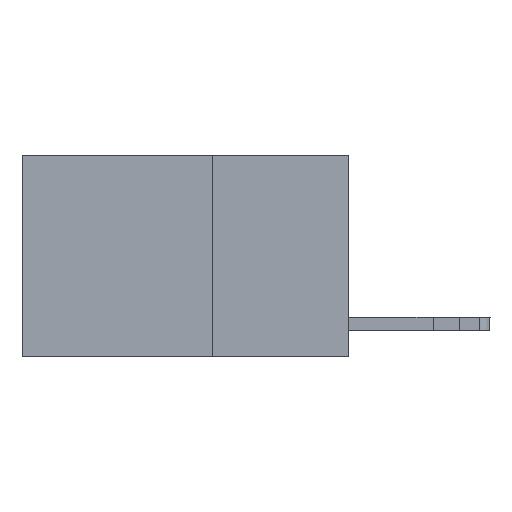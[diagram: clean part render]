
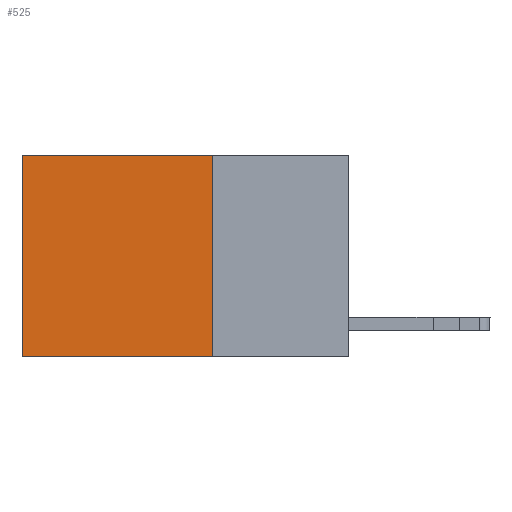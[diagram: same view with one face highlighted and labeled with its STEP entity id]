
A CAD part, left-side view. The second image highlights one B-rep face of the part: STEP entity #525.
In plain terms, the highlighted planar face has unit normal (-1, 0, 0).
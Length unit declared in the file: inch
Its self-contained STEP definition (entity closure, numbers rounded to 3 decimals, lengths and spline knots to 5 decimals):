
#215 = CARTESIAN_POINT ( 'NONE',  ( 0.2625, 0.6, -0.37 ) ) ;
#273 = VECTOR ( 'NONE', #13668, 39.37008 ) ;
#525 = ADVANCED_FACE ( 'NONE', ( #3201 ), #895, .F. ) ;
#894 = LINE ( 'NONE', #5625, #904 ) ;
#895 = PLANE ( 'NONE',  #9127 ) ;
#904 = VECTOR ( 'NONE', #4473, 39.37008 ) ;
#941 = EDGE_LOOP ( 'NONE', ( #10116, #12666, #1275, #1134 ) ) ;
#1053 = VERTEX_POINT ( 'NONE', #13430 ) ;
#1134 = ORIENTED_EDGE ( 'NONE', *, *, #11515, .T. ) ;
#1275 = ORIENTED_EDGE ( 'NONE', *, *, #5116, .F. ) ;
#1899 = CARTESIAN_POINT ( 'NONE',  ( 0.2625, 0.25, 0. ) ) ;
#3201 = FACE_OUTER_BOUND ( 'NONE', #941, .T. ) ;
#3376 = LINE ( 'NONE', #5924, #11583 ) ;
#3482 = VERTEX_POINT ( 'NONE', #215 ) ;
#3526 = EDGE_CURVE ( 'NONE', #1053, #3482, #3376, .T. ) ;
#4473 = DIRECTION ( 'NONE',  ( 0., 0., -1. ) ) ;
#5116 = EDGE_CURVE ( 'NONE', #12735, #12902, #894, .T. ) ;
#5625 = CARTESIAN_POINT ( 'NONE',  ( 0.2625, 0.25, 0. ) ) ;
#5765 = DIRECTION ( 'NONE',  ( 0., 0., -1. ) ) ;
#5924 = CARTESIAN_POINT ( 'NONE',  ( 0.2625, 0.6, 0. ) ) ;
#6502 = EDGE_CURVE ( 'NONE', #12902, #3482, #12560, .T. ) ;
#6607 = DIRECTION ( 'NONE',  ( 1., 0., 0. ) ) ;
#9127 = AXIS2_PLACEMENT_3D ( 'NONE', #1899, #6607, #5765 ) ;
#10116 = ORIENTED_EDGE ( 'NONE', *, *, #3526, .T. ) ;
#10122 = LINE ( 'NONE', #12528, #273 ) ;
#10482 = DIRECTION ( 'NONE',  ( 0., 0., -1. ) ) ;
#10710 = VECTOR ( 'NONE', #11104, 39.37008 ) ;
#11104 = DIRECTION ( 'NONE',  ( 0., 1., 0. ) ) ;
#11515 = EDGE_CURVE ( 'NONE', #12735, #1053, #10122, .T. ) ;
#11583 = VECTOR ( 'NONE', #10482, 39.37008 ) ;
#11749 = CARTESIAN_POINT ( 'NONE',  ( 0.2625, 0.25, -0.37 ) ) ;
#12528 = CARTESIAN_POINT ( 'NONE',  ( 0.2625, 0.25, 0. ) ) ;
#12560 = LINE ( 'NONE', #14941, #10710 ) ;
#12666 = ORIENTED_EDGE ( 'NONE', *, *, #6502, .F. ) ;
#12735 = VERTEX_POINT ( 'NONE', #14822 ) ;
#12902 = VERTEX_POINT ( 'NONE', #11749 ) ;
#13430 = CARTESIAN_POINT ( 'NONE',  ( 0.2625, 0.6, 0. ) ) ;
#13668 = DIRECTION ( 'NONE',  ( 0., 1., 0. ) ) ;
#14822 = CARTESIAN_POINT ( 'NONE',  ( 0.2625, 0.25, 0. ) ) ;
#14941 = CARTESIAN_POINT ( 'NONE',  ( 0.2625, 0.25, -0.37 ) ) ;
